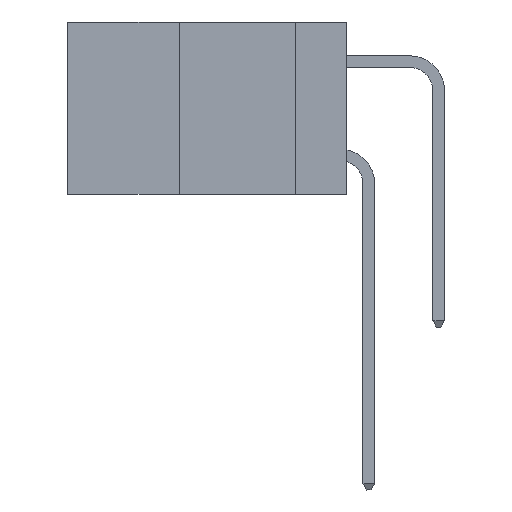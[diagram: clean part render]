
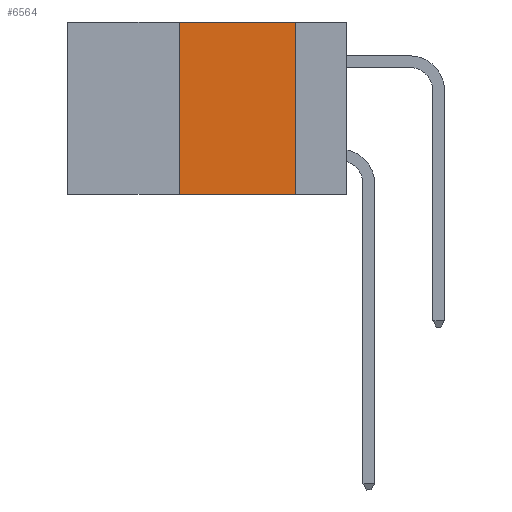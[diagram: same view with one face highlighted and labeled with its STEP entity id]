
A CAD part, left-side view. The second image highlights one B-rep face of the part: STEP entity #6564.
In plain terms, the highlighted planar face has unit normal (-1, 0, 0).
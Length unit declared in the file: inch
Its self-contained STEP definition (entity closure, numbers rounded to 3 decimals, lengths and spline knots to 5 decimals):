
#511 = EDGE_CURVE ( 'NONE', #11374, #5822, #12487, .T. ) ;
#924 = DIRECTION ( 'NONE',  ( 0., -1., 0. ) ) ;
#994 = CARTESIAN_POINT ( 'NONE',  ( 0., 0.11, 0. ) ) ;
#998 = CARTESIAN_POINT ( 'NONE',  ( 0., 0.6, -0.37 ) ) ;
#1458 = DIRECTION ( 'NONE',  ( 0., 0., -1. ) ) ;
#1484 = LINE ( 'NONE', #5619, #4244 ) ;
#1557 = CARTESIAN_POINT ( 'NONE',  ( 0., 0.36, 0. ) ) ;
#2785 = ORIENTED_EDGE ( 'NONE', *, *, #511, .T. ) ;
#3030 = VERTEX_POINT ( 'NONE', #1557 ) ;
#3134 = VECTOR ( 'NONE', #10018, 39.37008 ) ;
#4244 = VECTOR ( 'NONE', #14330, 39.37008 ) ;
#4738 = CARTESIAN_POINT ( 'NONE',  ( 0., 0.11, -0.37 ) ) ;
#5242 = EDGE_CURVE ( 'NONE', #6746, #5822, #13263, .T. ) ;
#5553 = CARTESIAN_POINT ( 'NONE',  ( 0., 0.6, 0. ) ) ;
#5619 = CARTESIAN_POINT ( 'NONE',  ( 0., 0.36, 0. ) ) ;
#5822 = VERTEX_POINT ( 'NONE', #4738 ) ;
#6107 = LINE ( 'NONE', #5553, #3134 ) ;
#6564 = ADVANCED_FACE ( 'NONE', ( #11086 ), #7153, .F. ) ;
#6746 = VERTEX_POINT ( 'NONE', #7436 ) ;
#7153 = PLANE ( 'NONE',  #12515 ) ;
#7436 = CARTESIAN_POINT ( 'NONE',  ( 0., 0.11, 0. ) ) ;
#7998 = EDGE_LOOP ( 'NONE', ( #9221, #9777, #9980, #2785 ) ) ;
#8231 = DIRECTION ( 'NONE',  ( 1., 0., 0. ) ) ;
#8864 = VECTOR ( 'NONE', #924, 39.37008 ) ;
#9221 = ORIENTED_EDGE ( 'NONE', *, *, #5242, .F. ) ;
#9777 = ORIENTED_EDGE ( 'NONE', *, *, #13688, .F. ) ;
#9980 = ORIENTED_EDGE ( 'NONE', *, *, #11062, .F. ) ;
#10018 = DIRECTION ( 'NONE',  ( 0., -1., 0. ) ) ;
#10410 = VECTOR ( 'NONE', #13848, 39.37008 ) ;
#10671 = CARTESIAN_POINT ( 'NONE',  ( 0., 0.36, -0.37 ) ) ;
#11062 = EDGE_CURVE ( 'NONE', #11374, #3030, #1484, .T. ) ;
#11086 = FACE_OUTER_BOUND ( 'NONE', #7998, .T. ) ;
#11374 = VERTEX_POINT ( 'NONE', #10671 ) ;
#11598 = CARTESIAN_POINT ( 'NONE',  ( 0., 0.6, 0. ) ) ;
#12487 = LINE ( 'NONE', #998, #8864 ) ;
#12515 = AXIS2_PLACEMENT_3D ( 'NONE', #11598, #8231, #1458 ) ;
#13263 = LINE ( 'NONE', #994, #10410 ) ;
#13688 = EDGE_CURVE ( 'NONE', #3030, #6746, #6107, .T. ) ;
#13848 = DIRECTION ( 'NONE',  ( 0., 0., -1. ) ) ;
#14330 = DIRECTION ( 'NONE',  ( 0., 0., 1. ) ) ;
